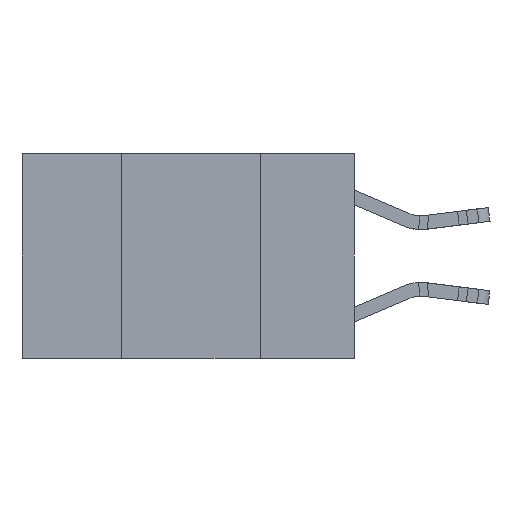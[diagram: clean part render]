
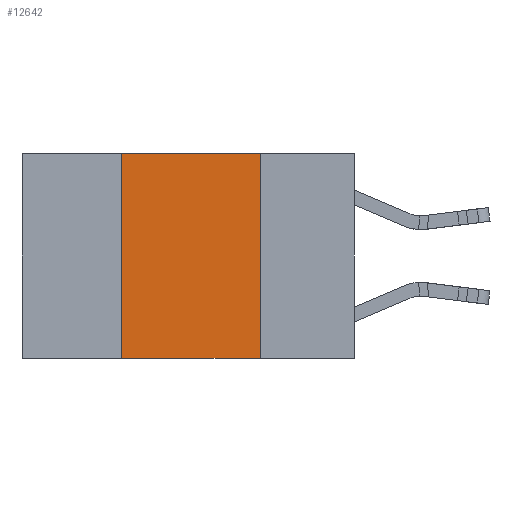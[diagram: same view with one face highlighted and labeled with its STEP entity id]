
A CAD part, left-side view. The second image highlights one B-rep face of the part: STEP entity #12642.
In plain terms, the highlighted planar face has unit normal (-1, 0, 0).
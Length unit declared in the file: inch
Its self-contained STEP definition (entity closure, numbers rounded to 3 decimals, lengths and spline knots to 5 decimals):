
#190 = ORIENTED_EDGE ( 'NONE', *, *, #3039, .F. ) ;
#986 = CARTESIAN_POINT ( 'NONE',  ( 0., 0.17, 0. ) ) ;
#1313 = CARTESIAN_POINT ( 'NONE',  ( 0., 0.6, 0. ) ) ;
#1743 = ORIENTED_EDGE ( 'NONE', *, *, #13764, .F. ) ;
#3039 = EDGE_CURVE ( 'NONE', #12856, #22417, #17729, .T. ) ;
#4172 = CARTESIAN_POINT ( 'NONE',  ( 0., 0.17, -0.37 ) ) ;
#4934 = LINE ( 'NONE', #16724, #21770 ) ;
#4941 = CARTESIAN_POINT ( 'NONE',  ( 0., 0.17, 0. ) ) ;
#5181 = ORIENTED_EDGE ( 'NONE', *, *, #23923, .F. ) ;
#5994 = CARTESIAN_POINT ( 'NONE',  ( 0., 0.42, -0.37 ) ) ;
#6564 = CARTESIAN_POINT ( 'NONE',  ( 0., 0.42, 0. ) ) ;
#6647 = DIRECTION ( 'NONE',  ( 0., 0., -1. ) ) ;
#9605 = FACE_OUTER_BOUND ( 'NONE', #28484, .T. ) ;
#11032 = DIRECTION ( 'NONE',  ( 0., -1., 0. ) ) ;
#11091 = VERTEX_POINT ( 'NONE', #5994 ) ;
#11225 = CARTESIAN_POINT ( 'NONE',  ( 0., 0.6, 0. ) ) ;
#12642 = ADVANCED_FACE ( 'NONE', ( #9605 ), #18531, .F. ) ;
#12820 = AXIS2_PLACEMENT_3D ( 'NONE', #11225, #20941, #6647 ) ;
#12856 = VERTEX_POINT ( 'NONE', #19242 ) ;
#13764 = EDGE_CURVE ( 'NONE', #11091, #12856, #17013, .T. ) ;
#14567 = ORIENTED_EDGE ( 'NONE', *, *, #15174, .T. ) ;
#15174 = EDGE_CURVE ( 'NONE', #11091, #29234, #4934, .T. ) ;
#16724 = CARTESIAN_POINT ( 'NONE',  ( 0., 0.6, -0.37 ) ) ;
#17011 = LINE ( 'NONE', #986, #22617 ) ;
#17013 = LINE ( 'NONE', #6564, #22619 ) ;
#17729 = LINE ( 'NONE', #1313, #29621 ) ;
#18531 = PLANE ( 'NONE',  #12820 ) ;
#19242 = CARTESIAN_POINT ( 'NONE',  ( 0., 0.42, 0. ) ) ;
#20239 = DIRECTION ( 'NONE',  ( 0., 0., -1. ) ) ;
#20941 = DIRECTION ( 'NONE',  ( 1., 0., 0. ) ) ;
#21770 = VECTOR ( 'NONE', #26100, 39.37008 ) ;
#22417 = VERTEX_POINT ( 'NONE', #4941 ) ;
#22617 = VECTOR ( 'NONE', #20239, 39.37008 ) ;
#22619 = VECTOR ( 'NONE', #28040, 39.37008 ) ;
#23923 = EDGE_CURVE ( 'NONE', #22417, #29234, #17011, .T. ) ;
#26100 = DIRECTION ( 'NONE',  ( 0., -1., 0. ) ) ;
#28040 = DIRECTION ( 'NONE',  ( 0., 0., 1. ) ) ;
#28484 = EDGE_LOOP ( 'NONE', ( #5181, #190, #1743, #14567 ) ) ;
#29234 = VERTEX_POINT ( 'NONE', #4172 ) ;
#29621 = VECTOR ( 'NONE', #11032, 39.37008 ) ;
